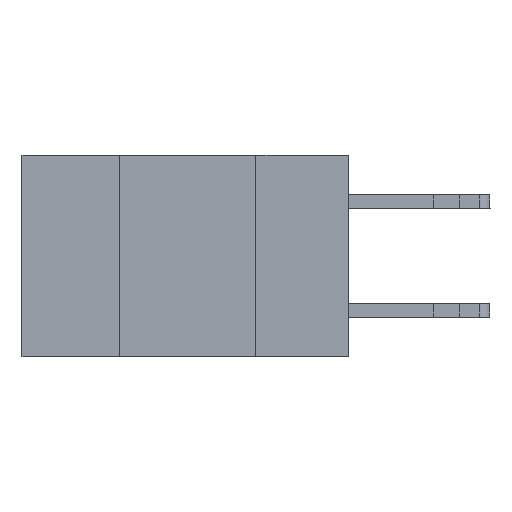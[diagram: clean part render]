
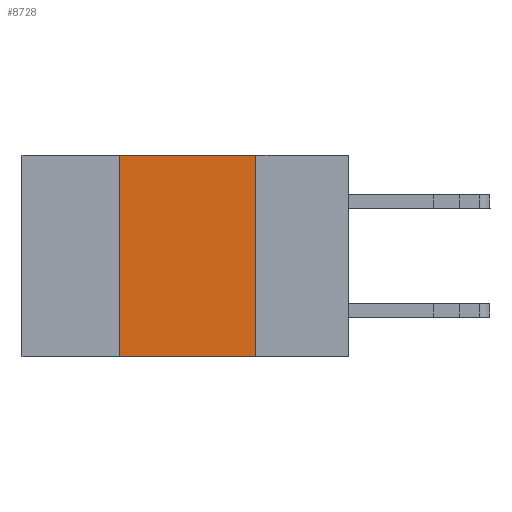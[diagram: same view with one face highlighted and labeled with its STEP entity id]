
A CAD part, left-side view. The second image highlights one B-rep face of the part: STEP entity #8728.
In plain terms, the highlighted planar face has unit normal (-1, 0, 0).
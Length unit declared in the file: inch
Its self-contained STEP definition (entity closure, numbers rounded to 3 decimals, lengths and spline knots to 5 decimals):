
#183 = PLANE ( 'NONE',  #19619 ) ;
#227 = ORIENTED_EDGE ( 'NONE', *, *, #21059, .T. ) ;
#1012 = LINE ( 'NONE', #10150, #18822 ) ;
#1054 = DIRECTION ( 'NONE',  ( 0., 0., -1. ) ) ;
#1519 = CARTESIAN_POINT ( 'NONE',  ( 0., 0.42, 0. ) ) ;
#1615 = FACE_OUTER_BOUND ( 'NONE', #1946, .T. ) ;
#1946 = EDGE_LOOP ( 'NONE', ( #3215, #12697, #17087, #227 ) ) ;
#2065 = DIRECTION ( 'NONE',  ( 0., 0., 1. ) ) ;
#3215 = ORIENTED_EDGE ( 'NONE', *, *, #18450, .F. ) ;
#3681 = VERTEX_POINT ( 'NONE', #4687 ) ;
#3700 = DIRECTION ( 'NONE',  ( 0., 0., -1. ) ) ;
#4084 = EDGE_CURVE ( 'NONE', #10890, #5205, #20850, .T. ) ;
#4687 = CARTESIAN_POINT ( 'NONE',  ( 0., 0.17, 0. ) ) ;
#5205 = VERTEX_POINT ( 'NONE', #1519 ) ;
#5913 = VECTOR ( 'NONE', #1054, 39.37008 ) ;
#6579 = LINE ( 'NONE', #15036, #14881 ) ;
#8728 = ADVANCED_FACE ( 'NONE', ( #1615 ), #183, .F. ) ;
#10150 = CARTESIAN_POINT ( 'NONE',  ( 0., 0.6, 0. ) ) ;
#10890 = VERTEX_POINT ( 'NONE', #17614 ) ;
#11337 = LINE ( 'NONE', #20981, #5913 ) ;
#12068 = CARTESIAN_POINT ( 'NONE',  ( 0., 0.6, 0. ) ) ;
#12697 = ORIENTED_EDGE ( 'NONE', *, *, #13175, .F. ) ;
#13175 = EDGE_CURVE ( 'NONE', #5205, #3681, #1012, .T. ) ;
#13741 = DIRECTION ( 'NONE',  ( 1., 0., 0. ) ) ;
#14444 = VERTEX_POINT ( 'NONE', #20935 ) ;
#14881 = VECTOR ( 'NONE', #16694, 39.37008 ) ;
#15036 = CARTESIAN_POINT ( 'NONE',  ( 0., 0.6, -0.37 ) ) ;
#16694 = DIRECTION ( 'NONE',  ( 0., -1., 0. ) ) ;
#17087 = ORIENTED_EDGE ( 'NONE', *, *, #4084, .F. ) ;
#17614 = CARTESIAN_POINT ( 'NONE',  ( 0., 0.42, -0.37 ) ) ;
#17620 = VECTOR ( 'NONE', #2065, 39.37008 ) ;
#18450 = EDGE_CURVE ( 'NONE', #3681, #14444, #11337, .T. ) ;
#18773 = CARTESIAN_POINT ( 'NONE',  ( 0., 0.42, 0. ) ) ;
#18822 = VECTOR ( 'NONE', #20898, 39.37008 ) ;
#19619 = AXIS2_PLACEMENT_3D ( 'NONE', #12068, #13741, #3700 ) ;
#20850 = LINE ( 'NONE', #18773, #17620 ) ;
#20898 = DIRECTION ( 'NONE',  ( 0., -1., 0. ) ) ;
#20935 = CARTESIAN_POINT ( 'NONE',  ( 0., 0.17, -0.37 ) ) ;
#20981 = CARTESIAN_POINT ( 'NONE',  ( 0., 0.17, 0. ) ) ;
#21059 = EDGE_CURVE ( 'NONE', #10890, #14444, #6579, .T. ) ;
